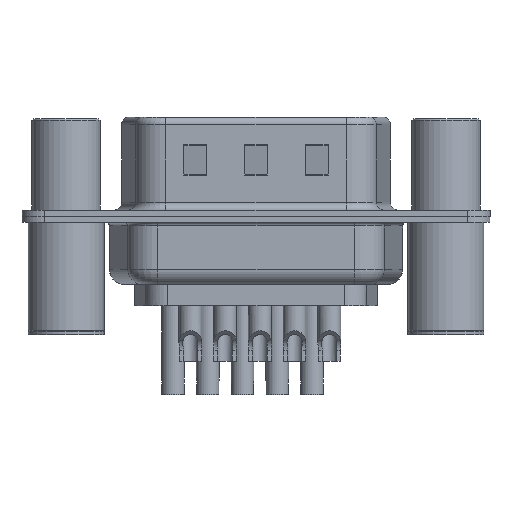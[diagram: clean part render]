
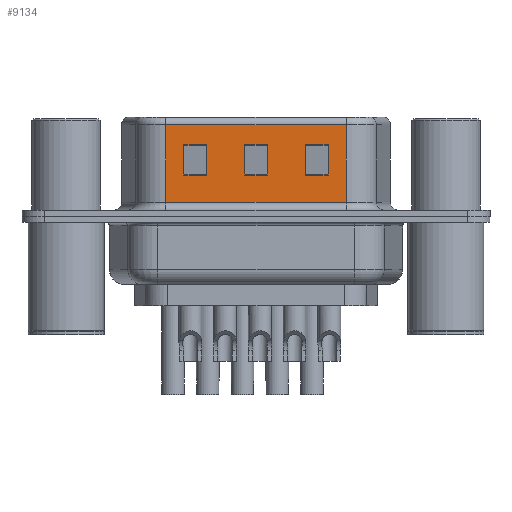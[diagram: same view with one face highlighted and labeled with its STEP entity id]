
A CAD part, front view. The second image highlights one B-rep face of the part: STEP entity #9134.
In plain terms, the highlighted planar face has unit normal (0, -1, 0).
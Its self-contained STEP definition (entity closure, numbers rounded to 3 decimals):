
#206 = EDGE_CURVE ( 'NONE', #3895, #12500, #15219, .T. ) ;
#365 = VECTOR ( 'NONE', #14339, 1000. ) ;
#443 = CARTESIAN_POINT ( 'NONE',  ( 7.75, -4.55, 2.705 ) ) ;
#479 = ORIENTED_EDGE ( 'NONE', *, *, #13266, .T. ) ;
#809 = LINE ( 'NONE', #9947, #365 ) ;
#1210 = DIRECTION ( 'NONE',  ( -1., 0., 0. ) ) ;
#1419 = VERTEX_POINT ( 'NONE', #18485 ) ;
#1621 = VECTOR ( 'NONE', #4492, 1000. ) ;
#1659 = VECTOR ( 'NONE', #16869, 1000. ) ;
#1824 = LINE ( 'NONE', #6900, #16675 ) ;
#1892 = EDGE_CURVE ( 'NONE', #4174, #3061, #3191, .T. ) ;
#2167 = CARTESIAN_POINT ( 'NONE',  ( 17.25, -4.55, 6.52 ) ) ;
#2169 = ORIENTED_EDGE ( 'NONE', *, *, #17080, .T. ) ;
#2302 = CARTESIAN_POINT ( 'NONE',  ( 13.25, -4.55, 4.705 ) ) ;
#2313 = VECTOR ( 'NONE', #3907, 1000. ) ;
#2332 = LINE ( 'NONE', #10223, #14313 ) ;
#2452 = CARTESIAN_POINT ( 'NONE',  ( 9.25, -4.55, 6.52 ) ) ;
#2623 = ORIENTED_EDGE ( 'NONE', *, *, #17796, .T. ) ;
#3019 = VERTEX_POINT ( 'NONE', #4439 ) ;
#3061 = VERTEX_POINT ( 'NONE', #16699 ) ;
#3191 = LINE ( 'NONE', #5894, #18071 ) ;
#3206 = EDGE_CURVE ( 'NONE', #12606, #13937, #8564, .T. ) ;
#3269 = ORIENTED_EDGE ( 'NONE', *, *, #11265, .T. ) ;
#3380 = FACE_OUTER_BOUND ( 'NONE', #16455, .T. ) ;
#3512 = VECTOR ( 'NONE', #9589, 1000. ) ;
#3688 = VECTOR ( 'NONE', #5208, 1000. ) ;
#3840 = LINE ( 'NONE', #15246, #11069 ) ;
#3895 = VERTEX_POINT ( 'NONE', #4239 ) ;
#3907 = DIRECTION ( 'NONE',  ( 0., 0., -1. ) ) ;
#3998 = CARTESIAN_POINT ( 'NONE',  ( 18.451, -4.55, 2.705 ) ) ;
#4174 = VERTEX_POINT ( 'NONE', #12450 ) ;
#4239 = CARTESIAN_POINT ( 'NONE',  ( 9.25, -4.55, 2.705 ) ) ;
#4435 = ORIENTED_EDGE ( 'NONE', *, *, #4756, .T. ) ;
#4439 = CARTESIAN_POINT ( 'NONE',  ( 11.75, -4.55, 4.705 ) ) ;
#4492 = DIRECTION ( 'NONE',  ( 0., 0., 1. ) ) ;
#4706 = VECTOR ( 'NONE', #5541, 1000. ) ;
#4756 = EDGE_CURVE ( 'NONE', #14139, #3019, #8863, .T. ) ;
#4790 = ORIENTED_EDGE ( 'NONE', *, *, #5670, .T. ) ;
#4818 = CARTESIAN_POINT ( 'NONE',  ( 14.451, -4.55, 2.705 ) ) ;
#4950 = VERTEX_POINT ( 'NONE', #2302 ) ;
#5194 = VECTOR ( 'NONE', #5691, 1000. ) ;
#5208 = DIRECTION ( 'NONE',  ( -1., 0., 0. ) ) ;
#5454 = DIRECTION ( 'NONE',  ( -1., 0., 0. ) ) ;
#5541 = DIRECTION ( 'NONE',  ( 0., 0., -1. ) ) ;
#5670 = EDGE_CURVE ( 'NONE', #15015, #3061, #9063, .T. ) ;
#5691 = DIRECTION ( 'NONE',  ( 1., 0., 0. ) ) ;
#5693 = EDGE_LOOP ( 'NONE', ( #3269, #8343, #2623, #4435 ) ) ;
#5798 = DIRECTION ( 'NONE',  ( 1., 0., 0. ) ) ;
#5862 = DIRECTION ( 'NONE',  ( 0., 0., -1. ) ) ;
#5874 = LINE ( 'NONE', #7131, #1621 ) ;
#5875 = EDGE_CURVE ( 'NONE', #12500, #10350, #5874, .T. ) ;
#5894 = CARTESIAN_POINT ( 'NONE',  ( 18.451, -4.55, 6.52 ) ) ;
#6537 = CARTESIAN_POINT ( 'NONE',  ( 14.451, -4.55, 4.705 ) ) ;
#6591 = ORIENTED_EDGE ( 'NONE', *, *, #5875, .T. ) ;
#6704 = PLANE ( 'NONE',  #13227 ) ;
#6745 = VERTEX_POINT ( 'NONE', #9126 ) ;
#6900 = CARTESIAN_POINT ( 'NONE',  ( 22.451, -4.55, 2.705 ) ) ;
#7131 = CARTESIAN_POINT ( 'NONE',  ( 7.75, -4.55, 6.52 ) ) ;
#7188 = FACE_BOUND ( 'NONE', #11755, .T. ) ;
#7238 = CARTESIAN_POINT ( 'NONE',  ( 18.451, -4.55, 4.705 ) ) ;
#7357 = VERTEX_POINT ( 'NONE', #16065 ) ;
#7638 = VECTOR ( 'NONE', #18100, 1000. ) ;
#7659 = FACE_BOUND ( 'NONE', #8147, .T. ) ;
#8021 = ORIENTED_EDGE ( 'NONE', *, *, #17072, .T. ) ;
#8147 = EDGE_LOOP ( 'NONE', ( #2169, #9929, #6591, #14875 ) ) ;
#8343 = ORIENTED_EDGE ( 'NONE', *, *, #13092, .T. ) ;
#8564 = LINE ( 'NONE', #2167, #4706 ) ;
#8571 = VERTEX_POINT ( 'NONE', #16946 ) ;
#8863 = LINE ( 'NONE', #12191, #1659 ) ;
#9063 = LINE ( 'NONE', #18507, #5194 ) ;
#9126 = CARTESIAN_POINT ( 'NONE',  ( 15.75, -4.55, 2.705 ) ) ;
#9134 = ADVANCED_FACE ( 'NONE', ( #7659, #7188, #15344, #3380 ), #6704, .F. ) ;
#9589 = DIRECTION ( 'NONE',  ( 0., 0., -1. ) ) ;
#9638 = DIRECTION ( 'NONE',  ( 0., 0., 1. ) ) ;
#9639 = EDGE_CURVE ( 'NONE', #10350, #8571, #15760, .T. ) ;
#9850 = EDGE_CURVE ( 'NONE', #13937, #6745, #1824, .T. ) ;
#9929 = ORIENTED_EDGE ( 'NONE', *, *, #206, .T. ) ;
#9947 = CARTESIAN_POINT ( 'NONE',  ( 6.549, -4.55, 6.52 ) ) ;
#9979 = LINE ( 'NONE', #2452, #2313 ) ;
#10180 = VECTOR ( 'NONE', #5454, 1000. ) ;
#10223 = CARTESIAN_POINT ( 'NONE',  ( 15.75, -4.55, 6.52 ) ) ;
#10309 = CARTESIAN_POINT ( 'NONE',  ( 6.549, -4.55, 6.02 ) ) ;
#10350 = VERTEX_POINT ( 'NONE', #18140 ) ;
#10643 = LINE ( 'NONE', #3998, #10180 ) ;
#10718 = VERTEX_POINT ( 'NONE', #10309 ) ;
#11069 = VECTOR ( 'NONE', #13787, 1000. ) ;
#11265 = EDGE_CURVE ( 'NONE', #3019, #4950, #12599, .T. ) ;
#11315 = ORIENTED_EDGE ( 'NONE', *, *, #9850, .T. ) ;
#11599 = CARTESIAN_POINT ( 'NONE',  ( 17.25, -4.55, 2.705 ) ) ;
#11713 = DIRECTION ( 'NONE',  ( 0., 0., 1. ) ) ;
#11755 = EDGE_LOOP ( 'NONE', ( #17898, #11315, #14051, #18384 ) ) ;
#12161 = VECTOR ( 'NONE', #5798, 1000. ) ;
#12191 = CARTESIAN_POINT ( 'NONE',  ( 11.75, -4.55, 6.52 ) ) ;
#12450 = CARTESIAN_POINT ( 'NONE',  ( 18.451, -4.55, 6.02 ) ) ;
#12500 = VERTEX_POINT ( 'NONE', #443 ) ;
#12599 = LINE ( 'NONE', #7238, #12161 ) ;
#12606 = VERTEX_POINT ( 'NONE', #13687 ) ;
#13092 = EDGE_CURVE ( 'NONE', #4950, #7357, #18392, .T. ) ;
#13227 = AXIS2_PLACEMENT_3D ( 'NONE', #16800, #18259, #9638 ) ;
#13266 = EDGE_CURVE ( 'NONE', #10718, #15015, #809, .T. ) ;
#13687 = CARTESIAN_POINT ( 'NONE',  ( 17.25, -4.55, 4.705 ) ) ;
#13787 = DIRECTION ( 'NONE',  ( 1., 0., 0. ) ) ;
#13828 = VECTOR ( 'NONE', #18285, 1000. ) ;
#13937 = VERTEX_POINT ( 'NONE', #11599 ) ;
#13961 = CARTESIAN_POINT ( 'NONE',  ( 18.451, -4.55, 6.02 ) ) ;
#14051 = ORIENTED_EDGE ( 'NONE', *, *, #14604, .T. ) ;
#14139 = VERTEX_POINT ( 'NONE', #16158 ) ;
#14290 = LINE ( 'NONE', #13961, #13828 ) ;
#14313 = VECTOR ( 'NONE', #11713, 1000. ) ;
#14339 = DIRECTION ( 'NONE',  ( 0., 0., -1. ) ) ;
#14604 = EDGE_CURVE ( 'NONE', #6745, #1419, #2332, .T. ) ;
#14875 = ORIENTED_EDGE ( 'NONE', *, *, #9639, .T. ) ;
#15015 = VERTEX_POINT ( 'NONE', #18265 ) ;
#15219 = LINE ( 'NONE', #4818, #3688 ) ;
#15246 = CARTESIAN_POINT ( 'NONE',  ( 22.451, -4.55, 4.705 ) ) ;
#15344 = FACE_BOUND ( 'NONE', #5693, .T. ) ;
#15760 = LINE ( 'NONE', #6537, #7638 ) ;
#16065 = CARTESIAN_POINT ( 'NONE',  ( 13.25, -4.55, 2.705 ) ) ;
#16158 = CARTESIAN_POINT ( 'NONE',  ( 11.75, -4.55, 2.705 ) ) ;
#16455 = EDGE_LOOP ( 'NONE', ( #16804, #8021, #479, #4790 ) ) ;
#16675 = VECTOR ( 'NONE', #1210, 1000. ) ;
#16699 = CARTESIAN_POINT ( 'NONE',  ( 18.451, -4.55, 0.9 ) ) ;
#16800 = CARTESIAN_POINT ( 'NONE',  ( 18.451, -4.55, 6.52 ) ) ;
#16804 = ORIENTED_EDGE ( 'NONE', *, *, #1892, .F. ) ;
#16869 = DIRECTION ( 'NONE',  ( 0., 0., 1. ) ) ;
#16946 = CARTESIAN_POINT ( 'NONE',  ( 9.25, -4.55, 4.705 ) ) ;
#17072 = EDGE_CURVE ( 'NONE', #4174, #10718, #14290, .T. ) ;
#17080 = EDGE_CURVE ( 'NONE', #8571, #3895, #9979, .T. ) ;
#17796 = EDGE_CURVE ( 'NONE', #7357, #14139, #10643, .T. ) ;
#17898 = ORIENTED_EDGE ( 'NONE', *, *, #3206, .T. ) ;
#18071 = VECTOR ( 'NONE', #5862, 1000. ) ;
#18100 = DIRECTION ( 'NONE',  ( 1., 0., 0. ) ) ;
#18140 = CARTESIAN_POINT ( 'NONE',  ( 7.75, -4.55, 4.705 ) ) ;
#18223 = CARTESIAN_POINT ( 'NONE',  ( 13.25, -4.55, 6.52 ) ) ;
#18259 = DIRECTION ( 'NONE',  ( 0., 1., 0. ) ) ;
#18265 = CARTESIAN_POINT ( 'NONE',  ( 6.549, -4.55, 0.9 ) ) ;
#18285 = DIRECTION ( 'NONE',  ( -1., 0., 0. ) ) ;
#18325 = EDGE_CURVE ( 'NONE', #1419, #12606, #3840, .T. ) ;
#18384 = ORIENTED_EDGE ( 'NONE', *, *, #18325, .T. ) ;
#18392 = LINE ( 'NONE', #18223, #3512 ) ;
#18485 = CARTESIAN_POINT ( 'NONE',  ( 15.75, -4.55, 4.705 ) ) ;
#18507 = CARTESIAN_POINT ( 'NONE',  ( 18.451, -4.55, 0.9 ) ) ;
